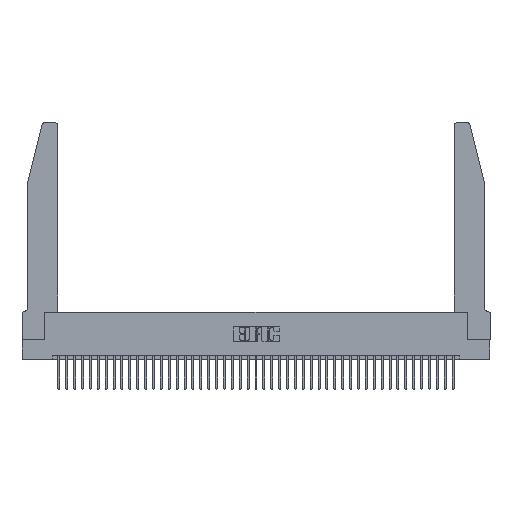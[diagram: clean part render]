
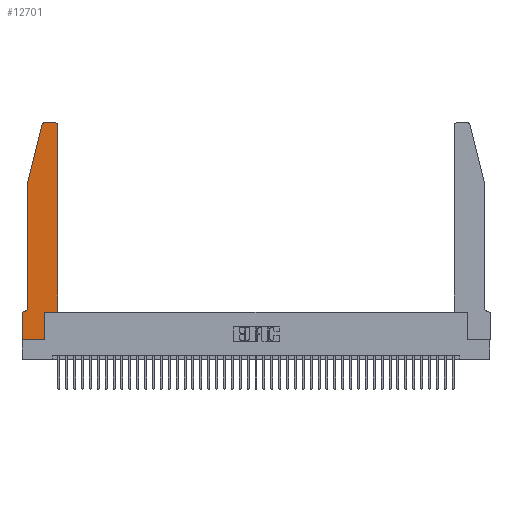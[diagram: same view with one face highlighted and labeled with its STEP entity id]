
A CAD part, top view. The second image highlights one B-rep face of the part: STEP entity #12701.
In plain terms, the highlighted planar face has unit normal (0, 0, 1).
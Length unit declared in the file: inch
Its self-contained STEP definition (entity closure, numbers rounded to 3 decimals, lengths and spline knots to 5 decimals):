
#46 = CARTESIAN_POINT ( 'NONE',  ( 0.2865, 0., 0.37 ) ) ;
#343 = LINE ( 'NONE', #41967, #17287 ) ;
#590 = ORIENTED_EDGE ( 'NONE', *, *, #14699, .T. ) ;
#1832 = EDGE_CURVE ( 'NONE', #15062, #25377, #42187, .T. ) ;
#1919 = ORIENTED_EDGE ( 'NONE', *, *, #16759, .T. ) ;
#2012 = CARTESIAN_POINT ( 'NONE',  ( 0.0755, 0.42, 0.37 ) ) ;
#2286 = EDGE_CURVE ( 'NONE', #16950, #20967, #33230, .T. ) ;
#2507 = VERTEX_POINT ( 'NONE', #13132 ) ;
#2552 = VECTOR ( 'NONE', #38347, 39.37008 ) ;
#2672 = CARTESIAN_POINT ( 'NONE',  ( 0.2605, 2.75, 0.37 ) ) ;
#4131 = CARTESIAN_POINT ( 'NONE',  ( 0.4205, 2.72, 0.37 ) ) ;
#4641 = LINE ( 'NONE', #7817, #29427 ) ;
#4907 = AXIS2_PLACEMENT_3D ( 'NONE', #4131, #27751, #7531 ) ;
#4987 = CARTESIAN_POINT ( 'NONE',  ( 0.284, 2.75, 0.37 ) ) ;
#5992 = ORIENTED_EDGE ( 'NONE', *, *, #8183, .T. ) ;
#6191 = CIRCLE ( 'NONE', #7851, 0.07 ) ;
#6641 = DIRECTION ( 'NONE',  ( 0., 1., 0. ) ) ;
#7239 = ORIENTED_EDGE ( 'NONE', *, *, #43149, .T. ) ;
#7412 = CARTESIAN_POINT ( 'NONE',  ( 0.25487, 2.72718, 0.37 ) ) ;
#7531 = DIRECTION ( 'NONE',  ( 1., 0., 0. ) ) ;
#7548 = CARTESIAN_POINT ( 'NONE',  ( 0.0755, 2., 0.37 ) ) ;
#7675 = PLANE ( 'NONE',  #18195 ) ;
#7817 = CARTESIAN_POINT ( 'NONE',  ( 0.4505, 0.35, 0.37 ) ) ;
#7851 = AXIS2_PLACEMENT_3D ( 'NONE', #38480, #18386, #41885 ) ;
#8183 = EDGE_CURVE ( 'NONE', #20967, #20220, #12152, .T. ) ;
#8919 = CARTESIAN_POINT ( 'NONE',  ( 0.2865, 0.35, 0.37 ) ) ;
#9279 = EDGE_CURVE ( 'NONE', #42693, #14816, #4641, .T. ) ;
#10974 = ORIENTED_EDGE ( 'NONE', *, *, #17399, .T. ) ;
#12031 = CARTESIAN_POINT ( 'NONE',  ( 0.4205, 2.75, 0.37 ) ) ;
#12152 = LINE ( 'NONE', #13874, #29010 ) ;
#12241 = CARTESIAN_POINT ( 'NONE',  ( 0.0755, 2., 0.37 ) ) ;
#12351 = VERTEX_POINT ( 'NONE', #26115 ) ;
#12701 = ADVANCED_FACE ( 'NONE', ( #39141 ), #7675, .T. ) ;
#13132 = CARTESIAN_POINT ( 'NONE',  ( 0.0755, 2., 0.37 ) ) ;
#13565 = ORIENTED_EDGE ( 'NONE', *, *, #9279, .T. ) ;
#13874 = CARTESIAN_POINT ( 'NONE',  ( 0., 0., 0.37 ) ) ;
#14443 = EDGE_CURVE ( 'NONE', #12351, #15062, #40063, .T. ) ;
#14480 = DIRECTION ( 'NONE',  ( 1., 0., 0. ) ) ;
#14699 = EDGE_CURVE ( 'NONE', #17267, #2507, #37464, .T. ) ;
#14816 = VERTEX_POINT ( 'NONE', #39666 ) ;
#15062 = VERTEX_POINT ( 'NONE', #12031 ) ;
#15361 = VECTOR ( 'NONE', #22261, 39.37008 ) ;
#15391 = DIRECTION ( 'NONE',  ( 0., 0., 1. ) ) ;
#15524 = CARTESIAN_POINT ( 'NONE',  ( 0.0755, 0.35, 0.37 ) ) ;
#15869 = CARTESIAN_POINT ( 'NONE',  ( 0.0055, 0.35, 0.37 ) ) ;
#16759 = EDGE_CURVE ( 'NONE', #20220, #19826, #21556, .T. ) ;
#16950 = VERTEX_POINT ( 'NONE', #15869 ) ;
#17129 = CARTESIAN_POINT ( 'NONE',  ( 0., 0.35, 0.37 ) ) ;
#17267 = VERTEX_POINT ( 'NONE', #7412 ) ;
#17287 = VECTOR ( 'NONE', #31994, 39.37008 ) ;
#17399 = EDGE_CURVE ( 'NONE', #25377, #17267, #40947, .T. ) ;
#18195 = AXIS2_PLACEMENT_3D ( 'NONE', #34617, #41359, #21216 ) ;
#18386 = DIRECTION ( 'NONE',  ( 0., 0., -1. ) ) ;
#19326 = ORIENTED_EDGE ( 'NONE', *, *, #33801, .T. ) ;
#19826 = VERTEX_POINT ( 'NONE', #46 ) ;
#20220 = VERTEX_POINT ( 'NONE', #22884 ) ;
#20967 = VERTEX_POINT ( 'NONE', #17129 ) ;
#21216 = DIRECTION ( 'NONE',  ( 1., 0., 0. ) ) ;
#21556 = LINE ( 'NONE', #34990, #2552 ) ;
#22261 = DIRECTION ( 'NONE',  ( -1., 0., 0. ) ) ;
#22880 = DIRECTION ( 'NONE',  ( -1., 0., 0. ) ) ;
#22884 = CARTESIAN_POINT ( 'NONE',  ( 0., 0., 0.37 ) ) ;
#24624 = ORIENTED_EDGE ( 'NONE', *, *, #31004, .T. ) ;
#25340 = AXIS2_PLACEMENT_3D ( 'NONE', #35512, #15391, #38859 ) ;
#25377 = VERTEX_POINT ( 'NONE', #4987 ) ;
#25400 = VECTOR ( 'NONE', #22880, 39.37008 ) ;
#26115 = CARTESIAN_POINT ( 'NONE',  ( 0.4505, 2.72, 0.37 ) ) ;
#27751 = DIRECTION ( 'NONE',  ( 0., 0., 1. ) ) ;
#27812 = VECTOR ( 'NONE', #6641, 39.37008 ) ;
#27907 = DIRECTION ( 'NONE',  ( 0., -1., 0. ) ) ;
#28776 = ORIENTED_EDGE ( 'NONE', *, *, #41092, .T. ) ;
#29010 = VECTOR ( 'NONE', #40720, 39.37008 ) ;
#29427 = VECTOR ( 'NONE', #14480, 39.37008 ) ;
#29644 = EDGE_LOOP ( 'NONE', ( #35153, #10974, #590, #7239, #28776, #34137, #5992, #1919, #24624, #13565, #19326, #42954 ) ) ;
#30652 = VECTOR ( 'NONE', #35773, 39.37008 ) ;
#31004 = EDGE_CURVE ( 'NONE', #19826, #42693, #343, .T. ) ;
#31324 = LINE ( 'NONE', #7548, #37094 ) ;
#31994 = DIRECTION ( 'NONE',  ( 0., 1., 0. ) ) ;
#33230 = LINE ( 'NONE', #15524, #15361 ) ;
#33587 = CARTESIAN_POINT ( 'NONE',  ( 0.4505, 0.35, 0.37 ) ) ;
#33801 = EDGE_CURVE ( 'NONE', #14816, #12351, #36702, .T. ) ;
#34137 = ORIENTED_EDGE ( 'NONE', *, *, #2286, .T. ) ;
#34617 = CARTESIAN_POINT ( 'NONE',  ( 0., 0.35, 0.37 ) ) ;
#34990 = CARTESIAN_POINT ( 'NONE',  ( 0., 0., 0.37 ) ) ;
#35153 = ORIENTED_EDGE ( 'NONE', *, *, #1832, .T. ) ;
#35512 = CARTESIAN_POINT ( 'NONE',  ( 0.284, 2.72, 0.37 ) ) ;
#35773 = DIRECTION ( 'NONE',  ( -0.239, -0.971, 0. ) ) ;
#36702 = LINE ( 'NONE', #33587, #27812 ) ;
#37094 = VECTOR ( 'NONE', #27907, 39.37008 ) ;
#37464 = LINE ( 'NONE', #12241, #30652 ) ;
#38347 = DIRECTION ( 'NONE',  ( 1., 0., 0. ) ) ;
#38480 = CARTESIAN_POINT ( 'NONE',  ( 0.0055, 0.42, 0.37 ) ) ;
#38859 = DIRECTION ( 'NONE',  ( 1., 0., 0. ) ) ;
#39141 = FACE_OUTER_BOUND ( 'NONE', #29644, .T. ) ;
#39666 = CARTESIAN_POINT ( 'NONE',  ( 0.4505, 0.35, 0.37 ) ) ;
#40063 = CIRCLE ( 'NONE', #4907, 0.03 ) ;
#40720 = DIRECTION ( 'NONE',  ( 0., -1., 0. ) ) ;
#40947 = CIRCLE ( 'NONE', #25340, 0.03 ) ;
#41092 = EDGE_CURVE ( 'NONE', #42096, #16950, #6191, .T. ) ;
#41359 = DIRECTION ( 'NONE',  ( 0., 0., 1. ) ) ;
#41885 = DIRECTION ( 'NONE',  ( -1., 0., 0. ) ) ;
#41967 = CARTESIAN_POINT ( 'NONE',  ( 0.2865, 0.35, 0.37 ) ) ;
#42096 = VERTEX_POINT ( 'NONE', #2012 ) ;
#42187 = LINE ( 'NONE', #2672, #25400 ) ;
#42693 = VERTEX_POINT ( 'NONE', #8919 ) ;
#42954 = ORIENTED_EDGE ( 'NONE', *, *, #14443, .T. ) ;
#43149 = EDGE_CURVE ( 'NONE', #2507, #42096, #31324, .T. ) ;
